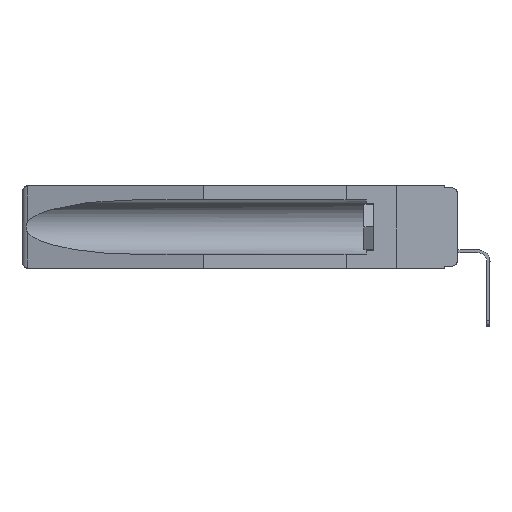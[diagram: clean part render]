
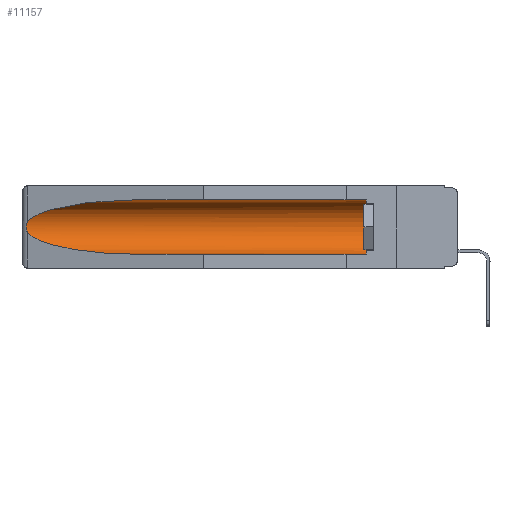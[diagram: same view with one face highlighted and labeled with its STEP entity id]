
A CAD part, left-side view. The second image highlights one B-rep face of the part: STEP entity #11157.
In plain terms, the highlighted cylindrical face has radius 2.857 mm (diameter 5.715 mm), a partial arc.
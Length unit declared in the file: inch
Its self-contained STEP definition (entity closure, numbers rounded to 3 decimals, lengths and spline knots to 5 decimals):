
#82 =( BOUNDED_CURVE ( )  B_SPLINE_CURVE ( 3, ( #965, #14468, #2873, #10399 ),
 .UNSPECIFIED., .F., .F. ) 
 B_SPLINE_CURVE_WITH_KNOTS ( ( 4, 4 ),
 ( 0.1948, 1.5708 ),
 .UNSPECIFIED. ) 
 CURVE ( )  GEOMETRIC_REPRESENTATION_ITEM ( )  RATIONAL_B_SPLINE_CURVE ( ( 1., 0.848, 0.848, 1. ) ) 
 REPRESENTATION_ITEM ( '' )  );
#965 = CARTESIAN_POINT ( 'NONE',  ( 0.26537, 1.52718, -0.19328 ) ) ;
#1238 = EDGE_CURVE ( 'NONE', #14068, #8863, #19114, .T. ) ;
#2101 = DIRECTION ( 'NONE',  ( 0., 1., 0. ) ) ;
#2484 = CARTESIAN_POINT ( 'NONE',  ( 0.155, 0.126, -0.059 ) ) ;
#2873 = CARTESIAN_POINT ( 'NONE',  ( 0.21114, 1.30732, -0.284 ) ) ;
#2974 = ORIENTED_EDGE ( 'NONE', *, *, #20039, .T. ) ;
#3103 = CARTESIAN_POINT ( 'NONE',  ( 0.155, -0.30754, -0.284 ) ) ;
#4417 = ORIENTED_EDGE ( 'NONE', *, *, #21001, .T. ) ;
#4460 =( BOUNDED_CURVE ( )  B_SPLINE_CURVE ( 3, ( #4497, #10368, #14107, #8309 ),
 .UNSPECIFIED., .F., .T. ) 
 B_SPLINE_CURVE_WITH_KNOTS ( ( 4, 4 ),
 ( 4.71239, 6.08839 ),
 .UNSPECIFIED. ) 
 CURVE ( )  GEOMETRIC_REPRESENTATION_ITEM ( )  RATIONAL_B_SPLINE_CURVE ( ( 1., 0.848, 0.848, 1. ) ) 
 REPRESENTATION_ITEM ( '' )  );
#4497 = CARTESIAN_POINT ( 'NONE',  ( 0.155, 1.07973, -0.059 ) ) ;
#4805 = VERTEX_POINT ( 'NONE', #12773 ) ;
#5205 = ORIENTED_EDGE ( 'NONE', *, *, #11412, .T. ) ;
#5859 = DIRECTION ( 'NONE',  ( 0., 0., 1. ) ) ;
#6496 = CARTESIAN_POINT ( 'NONE',  ( 0.26537, 1.52718, -0.14972 ) ) ;
#7009 = AXIS2_PLACEMENT_3D ( 'NONE', #15304, #17195, #5859 ) ;
#7977 = EDGE_CURVE ( 'NONE', #14068, #4805, #13098, .T. ) ;
#8235 = CARTESIAN_POINT ( 'NONE',  ( 0.26597, 1.52961, -0.15275 ) ) ;
#8309 = CARTESIAN_POINT ( 'NONE',  ( 0.26537, 1.52718, -0.14972 ) ) ;
#8468 = DIRECTION ( 'NONE',  ( 0., 1., 0. ) ) ;
#8863 = VERTEX_POINT ( 'NONE', #2484 ) ;
#9630 = CARTESIAN_POINT ( 'NONE',  ( 0.155, 0.126, -0.1715 ) ) ;
#10140 = CARTESIAN_POINT ( 'NONE',  ( 0.2673, 1.5327, -0.16383 ) ) ;
#10357 = ORIENTED_EDGE ( 'NONE', *, *, #20637, .T. ) ;
#10368 = CARTESIAN_POINT ( 'NONE',  ( 0.21114, 1.30732, -0.059 ) ) ;
#10399 = CARTESIAN_POINT ( 'NONE',  ( 0.155, 1.07973, -0.284 ) ) ;
#11156 = AXIS2_PLACEMENT_3D ( 'NONE', #9630, #21101, #13352 ) ;
#11157 = ADVANCED_FACE ( 'NONE', ( #20419 ), #11810, .F. ) ;
#11412 = EDGE_CURVE ( 'NONE', #11602, #11547, #4460, .T. ) ;
#11547 = VERTEX_POINT ( 'NONE', #16579 ) ;
#11602 = VERTEX_POINT ( 'NONE', #20180 ) ;
#11623 = CARTESIAN_POINT ( 'NONE',  ( 0.155, -0.30754, -0.059 ) ) ;
#11810 = CYLINDRICAL_SURFACE ( 'NONE', #7009, 0.1125 ) ;
#12378 = ORIENTED_EDGE ( 'NONE', *, *, #7977, .F. ) ;
#12443 = CARTESIAN_POINT ( 'NONE',  ( 0.2675, 1.53308, -0.16763 ) ) ;
#12773 = CARTESIAN_POINT ( 'NONE',  ( 0.155, 1.07973, -0.284 ) ) ;
#13098 = LINE ( 'NONE', #3103, #21450 ) ;
#13352 = DIRECTION ( 'NONE',  ( 0., 0., 1. ) ) ;
#13655 = CARTESIAN_POINT ( 'NONE',  ( 0.155, 0.126, -0.284 ) ) ;
#13737 = B_SPLINE_CURVE_WITH_KNOTS ( 'NONE', 3,
 ( #6496, #8235, #21535, #10140, #12443, #16580, #24024, #20101, #23847, #14517 ),
 .UNSPECIFIED., .F., .F.,
 ( 4, 2, 2, 2, 4 ),
 ( 0., 0.00029, 0.00058, 0.00087, 0.00117 ),
 .UNSPECIFIED. ) ;
#14068 = VERTEX_POINT ( 'NONE', #13655 ) ;
#14107 = CARTESIAN_POINT ( 'NONE',  ( 0.25451, 1.48313, -0.09465 ) ) ;
#14468 = CARTESIAN_POINT ( 'NONE',  ( 0.25451, 1.48313, -0.24835 ) ) ;
#14517 = CARTESIAN_POINT ( 'NONE',  ( 0.26537, 1.52718, -0.19328 ) ) ;
#15066 = LINE ( 'NONE', #11623, #15671 ) ;
#15304 = CARTESIAN_POINT ( 'NONE',  ( 0.155, -0.30754, -0.1715 ) ) ;
#15671 = VECTOR ( 'NONE', #2101, 39.37008 ) ;
#16319 = VERTEX_POINT ( 'NONE', #24213 ) ;
#16579 = CARTESIAN_POINT ( 'NONE',  ( 0.26537, 1.52718, -0.14972 ) ) ;
#16580 = CARTESIAN_POINT ( 'NONE',  ( 0.2675, 1.53308, -0.17534 ) ) ;
#17190 = EDGE_LOOP ( 'NONE', ( #5205, #10357, #2974, #12378, #23678, #4417 ) ) ;
#17195 = DIRECTION ( 'NONE',  ( 0., 1., 0. ) ) ;
#19114 = CIRCLE ( 'NONE', #11156, 0.1125 ) ;
#20039 = EDGE_CURVE ( 'NONE', #16319, #4805, #82, .T. ) ;
#20101 = CARTESIAN_POINT ( 'NONE',  ( 0.26655, 1.53094, -0.18657 ) ) ;
#20180 = CARTESIAN_POINT ( 'NONE',  ( 0.155, 1.07973, -0.059 ) ) ;
#20419 = FACE_OUTER_BOUND ( 'NONE', #17190, .T. ) ;
#20637 = EDGE_CURVE ( 'NONE', #11547, #16319, #13737, .T. ) ;
#21001 = EDGE_CURVE ( 'NONE', #8863, #11602, #15066, .T. ) ;
#21101 = DIRECTION ( 'NONE',  ( 0., -1., 0. ) ) ;
#21450 = VECTOR ( 'NONE', #8468, 39.37008 ) ;
#21535 = CARTESIAN_POINT ( 'NONE',  ( 0.26654, 1.53092, -0.15636 ) ) ;
#23678 = ORIENTED_EDGE ( 'NONE', *, *, #1238, .T. ) ;
#23847 = CARTESIAN_POINT ( 'NONE',  ( 0.26597, 1.5296, -0.19026 ) ) ;
#24024 = CARTESIAN_POINT ( 'NONE',  ( 0.2673, 1.53269, -0.17917 ) ) ;
#24213 = CARTESIAN_POINT ( 'NONE',  ( 0.26537, 1.52718, -0.19328 ) ) ;
